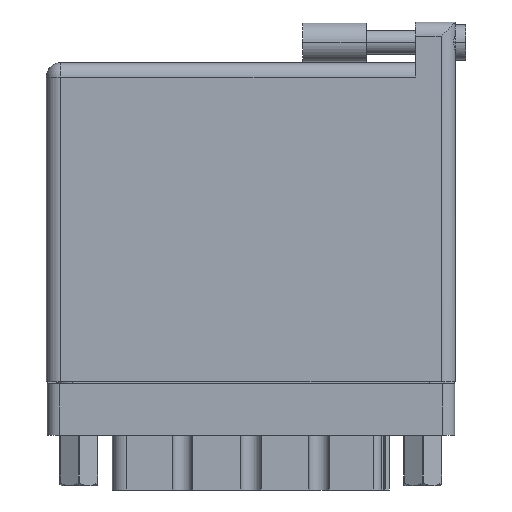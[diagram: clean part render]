
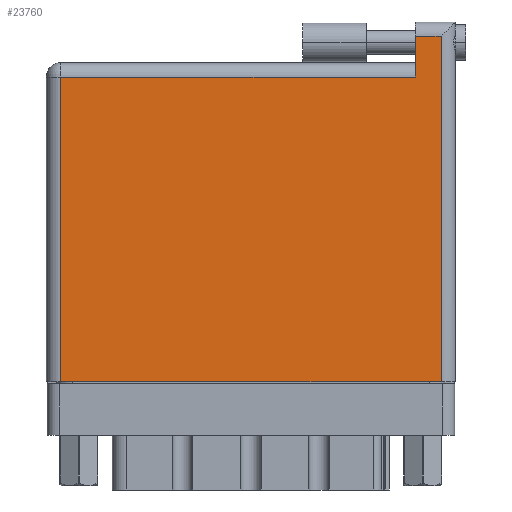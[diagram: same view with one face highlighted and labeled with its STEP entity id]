
A CAD part, front view. The second image highlights one B-rep face of the part: STEP entity #23760.
In plain terms, the highlighted face is planar.
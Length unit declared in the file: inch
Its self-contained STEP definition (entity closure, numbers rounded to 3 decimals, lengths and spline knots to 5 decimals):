
#95 = DIRECTION ( 'NONE',  ( -1., 0., 0. ) ) ;
#1062 = LINE ( 'NONE', #7006, #43126 ) ;
#1440 = VECTOR ( 'NONE', #14918, 39.37008 ) ;
#1631 = ORIENTED_EDGE ( 'NONE', *, *, #41435, .T. ) ;
#1813 = VECTOR ( 'NONE', #36834, 39.37008 ) ;
#1970 = CARTESIAN_POINT ( 'NONE',  ( 1.938, 1.766, 0. ) ) ;
#2269 = DIRECTION ( 'NONE',  ( 0., -1., 0. ) ) ;
#4203 = CARTESIAN_POINT ( 'NONE',  ( 0.07, 0., 0. ) ) ;
#5115 = CARTESIAN_POINT ( 'NONE',  ( 1.811, 1.766, 0. ) ) ;
#7006 = CARTESIAN_POINT ( 'NONE',  ( 0., 1.696, 0. ) ) ;
#7388 = EDGE_CURVE ( 'NONE', #30413, #25045, #41248, .T. ) ;
#7830 = VECTOR ( 'NONE', #12650, 39.37008 ) ;
#7887 = CARTESIAN_POINT ( 'NONE',  ( 1.938, 0., 0. ) ) ;
#11803 = LINE ( 'NONE', #5115, #1813 ) ;
#12005 = DIRECTION ( 'NONE',  ( 1., 0., 0. ) ) ;
#12650 = DIRECTION ( 'NONE',  ( 0., 1., 0. ) ) ;
#14918 = DIRECTION ( 'NONE',  ( -1., 0., 0. ) ) ;
#15424 = CARTESIAN_POINT ( 'NONE',  ( 0., 0., 0. ) ) ;
#16685 = ORIENTED_EDGE ( 'NONE', *, *, #7388, .T. ) ;
#17239 = LINE ( 'NONE', #1970, #7830 ) ;
#17698 = CARTESIAN_POINT ( 'NONE',  ( 0.07, 1.496, 0. ) ) ;
#17849 = VERTEX_POINT ( 'NONE', #7887 ) ;
#21008 = CARTESIAN_POINT ( 'NONE',  ( 0., 1.566, 0. ) ) ;
#21303 = PLANE ( 'NONE',  #27963 ) ;
#21872 = EDGE_CURVE ( 'NONE', #17849, #41617, #17239, .T. ) ;
#23760 = ADVANCED_FACE ( 'NONE', ( #25351 ), #21303, .F. ) ;
#25045 = VERTEX_POINT ( 'NONE', #17698 ) ;
#25250 = CARTESIAN_POINT ( 'NONE',  ( 1.938, 1.696, 0. ) ) ;
#25351 = FACE_OUTER_BOUND ( 'NONE', #41716, .T. ) ;
#25881 = VERTEX_POINT ( 'NONE', #43352 ) ;
#27963 = AXIS2_PLACEMENT_3D ( 'NONE', #21008, #42472, #95 ) ;
#28565 = ORIENTED_EDGE ( 'NONE', *, *, #35637, .T. ) ;
#28653 = VECTOR ( 'NONE', #12005, 39.37008 ) ;
#30321 = ORIENTED_EDGE ( 'NONE', *, *, #37405, .T. ) ;
#30413 = VERTEX_POINT ( 'NONE', #39950 ) ;
#30418 = CARTESIAN_POINT ( 'NONE',  ( 0.07, 0., 0. ) ) ;
#31603 = CARTESIAN_POINT ( 'NONE',  ( 0., 1.496, 0. ) ) ;
#33716 = VERTEX_POINT ( 'NONE', #4203 ) ;
#34890 = ORIENTED_EDGE ( 'NONE', *, *, #36776, .T. ) ;
#35637 = EDGE_CURVE ( 'NONE', #33716, #17849, #44660, .T. ) ;
#36776 = EDGE_CURVE ( 'NONE', #25045, #33716, #37355, .T. ) ;
#36834 = DIRECTION ( 'NONE',  ( 0., -1., 0. ) ) ;
#37355 = LINE ( 'NONE', #30418, #41205 ) ;
#37405 = EDGE_CURVE ( 'NONE', #25881, #30413, #11803, .T. ) ;
#38961 = DIRECTION ( 'NONE',  ( -1., 0., 0. ) ) ;
#38967 = ORIENTED_EDGE ( 'NONE', *, *, #21872, .T. ) ;
#39950 = CARTESIAN_POINT ( 'NONE',  ( 1.811, 1.496, 0. ) ) ;
#41205 = VECTOR ( 'NONE', #2269, 39.37008 ) ;
#41248 = LINE ( 'NONE', #31603, #1440 ) ;
#41435 = EDGE_CURVE ( 'NONE', #41617, #25881, #1062, .T. ) ;
#41617 = VERTEX_POINT ( 'NONE', #25250 ) ;
#41716 = EDGE_LOOP ( 'NONE', ( #28565, #38967, #1631, #30321, #16685, #34890 ) ) ;
#42472 = DIRECTION ( 'NONE',  ( 0., 0., -1. ) ) ;
#43126 = VECTOR ( 'NONE', #38961, 39.37008 ) ;
#43352 = CARTESIAN_POINT ( 'NONE',  ( 1.811, 1.696, 0. ) ) ;
#44660 = LINE ( 'NONE', #15424, #28653 ) ;
